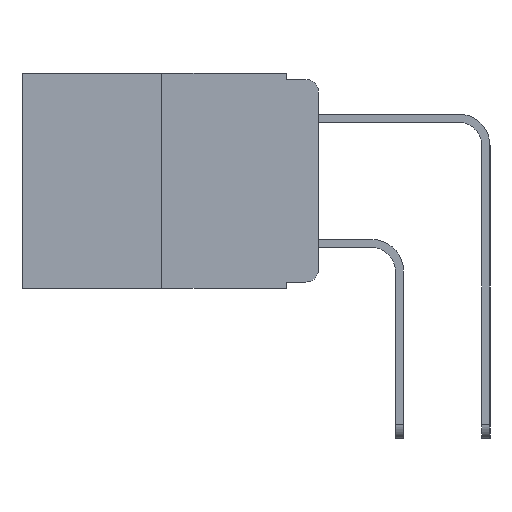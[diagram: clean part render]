
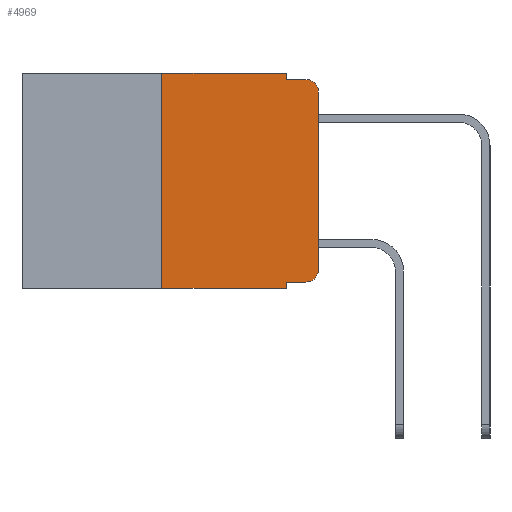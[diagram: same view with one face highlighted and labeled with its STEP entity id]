
A CAD part, left-side view. The second image highlights one B-rep face of the part: STEP entity #4969.
In plain terms, the highlighted planar face has unit normal (-1, 0, 0).
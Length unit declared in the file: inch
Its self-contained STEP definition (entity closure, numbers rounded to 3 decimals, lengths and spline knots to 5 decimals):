
#106 = VECTOR ( 'NONE', #17012, 39.37008 ) ;
#184 = EDGE_CURVE ( 'NONE', #19189, #13970, #19087, .T. ) ;
#607 = ORIENTED_EDGE ( 'NONE', *, *, #184, .F. ) ;
#1069 = EDGE_CURVE ( 'NONE', #5519, #13970, #20351, .T. ) ;
#1330 = EDGE_CURVE ( 'NONE', #5519, #19067, #20100, .T. ) ;
#2262 = DIRECTION ( 'NONE',  ( 0., 0., 1. ) ) ;
#2290 = CARTESIAN_POINT ( 'NONE',  ( 0., 0.473, 0. ) ) ;
#3207 = LINE ( 'NONE', #7459, #15558 ) ;
#3351 = CARTESIAN_POINT ( 'NONE',  ( 0., 0.051, 0. ) ) ;
#3535 = LINE ( 'NONE', #4221, #106 ) ;
#3569 = EDGE_CURVE ( 'NONE', #18475, #15763, #8952, .T. ) ;
#3956 = DIRECTION ( 'NONE',  ( 1., 0., 0. ) ) ;
#4125 = CARTESIAN_POINT ( 'NONE',  ( 0., 0.25, 0. ) ) ;
#4202 = CARTESIAN_POINT ( 'NONE',  ( 0., 0.051, -0.343 ) ) ;
#4221 = CARTESIAN_POINT ( 'NONE',  ( 0., 0.051, -0.333 ) ) ;
#4484 = ORIENTED_EDGE ( 'NONE', *, *, #13940, .F. ) ;
#4671 = EDGE_CURVE ( 'NONE', #15763, #7898, #17078, .T. ) ;
#4969 = ADVANCED_FACE ( 'NONE', ( #7858 ), #13632, .F. ) ;
#5320 = CARTESIAN_POINT ( 'NONE',  ( 0., 0.02, -0.313 ) ) ;
#5519 = VERTEX_POINT ( 'NONE', #9075 ) ;
#5738 = EDGE_CURVE ( 'NONE', #20717, #7898, #13416, .T. ) ;
#6212 = ORIENTED_EDGE ( 'NONE', *, *, #1069, .T. ) ;
#6637 = DIRECTION ( 'NONE',  ( 0., 0., -1. ) ) ;
#6737 = AXIS2_PLACEMENT_3D ( 'NONE', #19118, #9694, #20660 ) ;
#6950 = DIRECTION ( 'NONE',  ( 0., 0., -1. ) ) ;
#7043 = CARTESIAN_POINT ( 'NONE',  ( 0., 0.051, 0. ) ) ;
#7131 = EDGE_LOOP ( 'NONE', ( #9298, #8837, #8964, #12489, #4484, #10942, #6212, #607, #20139, #12661 ) ) ;
#7459 = CARTESIAN_POINT ( 'NONE',  ( 0., 0.473, 0. ) ) ;
#7609 = CARTESIAN_POINT ( 'NONE',  ( 0., 0.25, 0. ) ) ;
#7858 = FACE_OUTER_BOUND ( 'NONE', #7131, .T. ) ;
#7898 = VERTEX_POINT ( 'NONE', #17969 ) ;
#7932 = EDGE_CURVE ( 'NONE', #16010, #20717, #8719, .T. ) ;
#8012 = CARTESIAN_POINT ( 'NONE',  ( 0., 0., -0.03 ) ) ;
#8719 = LINE ( 'NONE', #19569, #12492 ) ;
#8837 = ORIENTED_EDGE ( 'NONE', *, *, #5738, .T. ) ;
#8952 = LINE ( 'NONE', #7043, #16881 ) ;
#8964 = ORIENTED_EDGE ( 'NONE', *, *, #4671, .F. ) ;
#9036 = CARTESIAN_POINT ( 'NONE',  ( 0., 0.051, 0. ) ) ;
#9075 = CARTESIAN_POINT ( 'NONE',  ( 0., 0.25, -0.343 ) ) ;
#9087 = DIRECTION ( 'NONE',  ( 0., -1., 0. ) ) ;
#9298 = ORIENTED_EDGE ( 'NONE', *, *, #7932, .T. ) ;
#9694 = DIRECTION ( 'NONE',  ( -1., 0., 0. ) ) ;
#9942 = CARTESIAN_POINT ( 'NONE',  ( 0., 0.473, -0.343 ) ) ;
#10942 = ORIENTED_EDGE ( 'NONE', *, *, #1330, .F. ) ;
#11187 = AXIS2_PLACEMENT_3D ( 'NONE', #2290, #3956, #15214 ) ;
#11527 = VECTOR ( 'NONE', #13873, 39.37008 ) ;
#12489 = ORIENTED_EDGE ( 'NONE', *, *, #3569, .F. ) ;
#12492 = VECTOR ( 'NONE', #18039, 39.37008 ) ;
#12661 = ORIENTED_EDGE ( 'NONE', *, *, #18923, .T. ) ;
#12934 = VECTOR ( 'NONE', #17585, 39.37008 ) ;
#13035 = CARTESIAN_POINT ( 'NONE',  ( 0., 0., -0.313 ) ) ;
#13416 = CIRCLE ( 'NONE', #6737, 0.02 ) ;
#13632 = PLANE ( 'NONE',  #11187 ) ;
#13697 = CARTESIAN_POINT ( 'NONE',  ( 0., 0.02, -0.333 ) ) ;
#13873 = DIRECTION ( 'NONE',  ( 0., -1., 0. ) ) ;
#13940 = EDGE_CURVE ( 'NONE', #19067, #18475, #3207, .T. ) ;
#13970 = VERTEX_POINT ( 'NONE', #4202 ) ;
#14408 = CARTESIAN_POINT ( 'NONE',  ( 0., 0.051, -0.01 ) ) ;
#15128 = DIRECTION ( 'NONE',  ( 0., 0., -1. ) ) ;
#15157 = VERTEX_POINT ( 'NONE', #13697 ) ;
#15214 = DIRECTION ( 'NONE',  ( 0., 0., -1. ) ) ;
#15558 = VECTOR ( 'NONE', #9087, 39.37008 ) ;
#15675 = CIRCLE ( 'NONE', #17347, 0.02 ) ;
#15763 = VERTEX_POINT ( 'NONE', #19881 ) ;
#16003 = VECTOR ( 'NONE', #2262, 39.37008 ) ;
#16010 = VERTEX_POINT ( 'NONE', #13035 ) ;
#16514 = DIRECTION ( 'NONE',  ( -1., 0., 0. ) ) ;
#16881 = VECTOR ( 'NONE', #15128, 39.37008 ) ;
#17012 = DIRECTION ( 'NONE',  ( 0., -1., 0. ) ) ;
#17078 = LINE ( 'NONE', #14408, #12934 ) ;
#17347 = AXIS2_PLACEMENT_3D ( 'NONE', #5320, #16514, #6950 ) ;
#17585 = DIRECTION ( 'NONE',  ( 0., -1., 0. ) ) ;
#17969 = CARTESIAN_POINT ( 'NONE',  ( 0., 0.02, -0.01 ) ) ;
#18039 = DIRECTION ( 'NONE',  ( 0., 0., 1. ) ) ;
#18475 = VERTEX_POINT ( 'NONE', #9036 ) ;
#18608 = VECTOR ( 'NONE', #6637, 39.37008 ) ;
#18923 = EDGE_CURVE ( 'NONE', #15157, #16010, #15675, .T. ) ;
#19067 = VERTEX_POINT ( 'NONE', #4125 ) ;
#19087 = LINE ( 'NONE', #3351, #18608 ) ;
#19118 = CARTESIAN_POINT ( 'NONE',  ( 0., 0.02, -0.03 ) ) ;
#19189 = VERTEX_POINT ( 'NONE', #20265 ) ;
#19569 = CARTESIAN_POINT ( 'NONE',  ( 0., 0., 0. ) ) ;
#19881 = CARTESIAN_POINT ( 'NONE',  ( 0., 0.051, -0.01 ) ) ;
#19956 = EDGE_CURVE ( 'NONE', #19189, #15157, #3535, .T. ) ;
#20100 = LINE ( 'NONE', #7609, #16003 ) ;
#20139 = ORIENTED_EDGE ( 'NONE', *, *, #19956, .T. ) ;
#20265 = CARTESIAN_POINT ( 'NONE',  ( 0., 0.051, -0.333 ) ) ;
#20351 = LINE ( 'NONE', #9942, #11527 ) ;
#20660 = DIRECTION ( 'NONE',  ( 0., 0., -1. ) ) ;
#20717 = VERTEX_POINT ( 'NONE', #8012 ) ;
